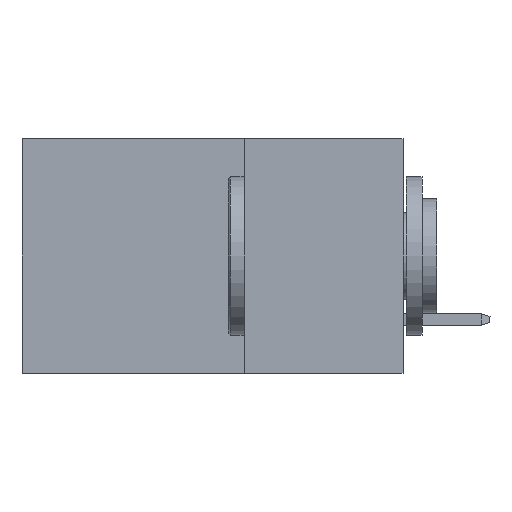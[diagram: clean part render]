
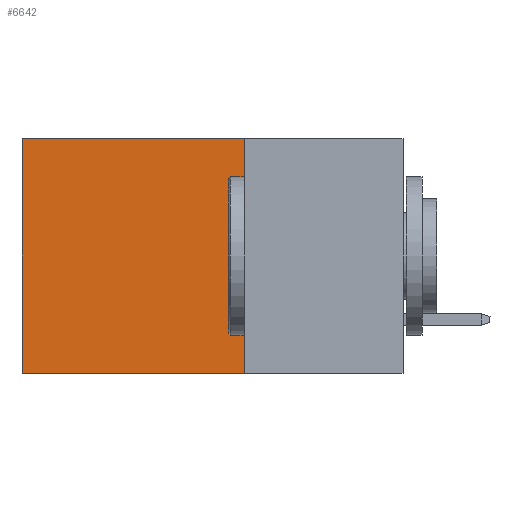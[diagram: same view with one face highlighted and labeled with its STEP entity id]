
A CAD part, left-side view. The second image highlights one B-rep face of the part: STEP entity #6642.
In plain terms, the highlighted planar face has unit normal (-1, 0, 0).
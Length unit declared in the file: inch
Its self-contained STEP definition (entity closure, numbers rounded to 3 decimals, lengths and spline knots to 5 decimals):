
#206 = CARTESIAN_POINT ( 'NONE',  ( 0.2875, 0.6, 0. ) ) ;
#350 = LINE ( 'NONE', #7649, #5644 ) ;
#702 = LINE ( 'NONE', #7334, #4569 ) ;
#740 = VECTOR ( 'NONE', #2437, 39.37008 ) ;
#954 = VECTOR ( 'NONE', #7240, 39.37008 ) ;
#1422 = CARTESIAN_POINT ( 'NONE',  ( 0.2875, 0.25, 0. ) ) ;
#1434 = VERTEX_POINT ( 'NONE', #5994 ) ;
#1671 = VERTEX_POINT ( 'NONE', #1422 ) ;
#1821 = CARTESIAN_POINT ( 'NONE',  ( 0.2875, 0.25, 0. ) ) ;
#1854 = CARTESIAN_POINT ( 'NONE',  ( 0.2875, 0.6, -0.37 ) ) ;
#2437 = DIRECTION ( 'NONE',  ( 0., 0., -1. ) ) ;
#3019 = FACE_OUTER_BOUND ( 'NONE', #7568, .T. ) ;
#3070 = VERTEX_POINT ( 'NONE', #1854 ) ;
#3143 = EDGE_CURVE ( 'NONE', #1434, #3070, #3435, .T. ) ;
#3435 = LINE ( 'NONE', #7942, #954 ) ;
#4569 = VECTOR ( 'NONE', #8770, 39.37008 ) ;
#4821 = ORIENTED_EDGE ( 'NONE', *, *, #9253, .F. ) ;
#5644 = VECTOR ( 'NONE', #6945, 39.37008 ) ;
#5898 = ORIENTED_EDGE ( 'NONE', *, *, #3143, .F. ) ;
#5923 = ORIENTED_EDGE ( 'NONE', *, *, #8555, .T. ) ;
#5968 = DIRECTION ( 'NONE',  ( 0., 0., -1. ) ) ;
#5994 = CARTESIAN_POINT ( 'NONE',  ( 0.2875, 0.25, -0.37 ) ) ;
#6642 = ADVANCED_FACE ( 'NONE', ( #3019 ), #6783, .F. ) ;
#6783 = PLANE ( 'NONE',  #8693 ) ;
#6945 = DIRECTION ( 'NONE',  ( 0., 1., 0. ) ) ;
#7134 = ORIENTED_EDGE ( 'NONE', *, *, #7280, .T. ) ;
#7240 = DIRECTION ( 'NONE',  ( 0., 1., 0. ) ) ;
#7280 = EDGE_CURVE ( 'NONE', #7330, #3070, #702, .T. ) ;
#7330 = VERTEX_POINT ( 'NONE', #206 ) ;
#7334 = CARTESIAN_POINT ( 'NONE',  ( 0.2875, 0.6, 0. ) ) ;
#7568 = EDGE_LOOP ( 'NONE', ( #7134, #5898, #4821, #5923 ) ) ;
#7649 = CARTESIAN_POINT ( 'NONE',  ( 0.2875, 0.25, 0. ) ) ;
#7942 = CARTESIAN_POINT ( 'NONE',  ( 0.2875, 0.25, -0.37 ) ) ;
#8555 = EDGE_CURVE ( 'NONE', #1671, #7330, #350, .T. ) ;
#8693 = AXIS2_PLACEMENT_3D ( 'NONE', #8980, #8840, #5968 ) ;
#8770 = DIRECTION ( 'NONE',  ( 0., 0., -1. ) ) ;
#8840 = DIRECTION ( 'NONE',  ( 1., 0., 0. ) ) ;
#8980 = CARTESIAN_POINT ( 'NONE',  ( 0.2875, 0.25, 0. ) ) ;
#9026 = LINE ( 'NONE', #1821, #740 ) ;
#9253 = EDGE_CURVE ( 'NONE', #1671, #1434, #9026, .T. ) ;
